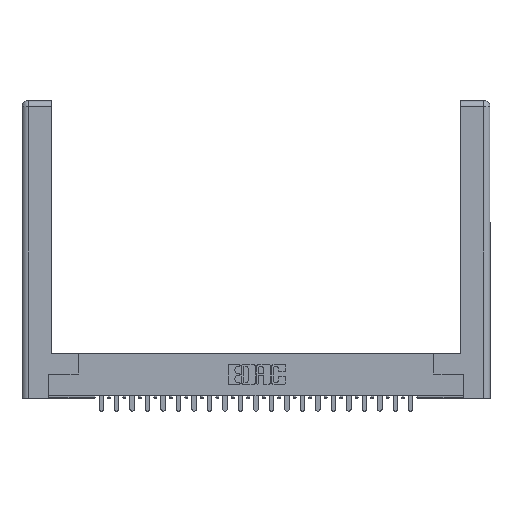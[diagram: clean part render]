
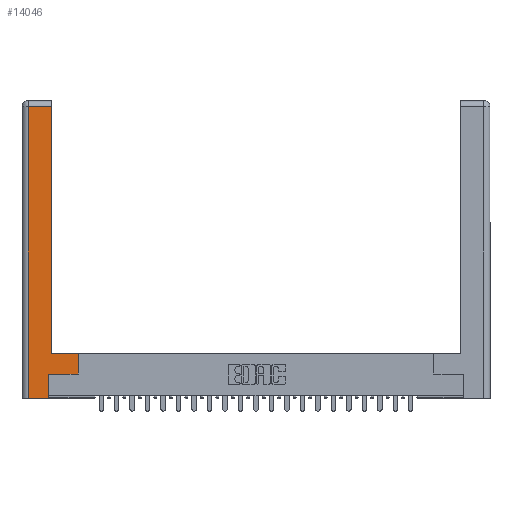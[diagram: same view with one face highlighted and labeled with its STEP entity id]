
A CAD part, top view. The second image highlights one B-rep face of the part: STEP entity #14046.
In plain terms, the highlighted planar face has unit normal (0, 0, 1).
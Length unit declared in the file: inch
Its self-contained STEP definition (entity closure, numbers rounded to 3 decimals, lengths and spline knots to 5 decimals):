
#110 = CARTESIAN_POINT ( 'NONE',  ( 0.265, 0., 0. ) ) ;
#806 = CARTESIAN_POINT ( 'NONE',  ( 0.295, 0.45, 0. ) ) ;
#1246 = ORIENTED_EDGE ( 'NONE', *, *, #8433, .T. ) ;
#1459 = DIRECTION ( 'NONE',  ( 0., 1., 0. ) ) ;
#1823 = VECTOR ( 'NONE', #17941, 39.37008 ) ;
#2029 = EDGE_CURVE ( 'NONE', #27252, #5921, #13883, .T. ) ;
#2467 = EDGE_CURVE ( 'NONE', #15852, #5702, #19233, .T. ) ;
#2565 = VECTOR ( 'NONE', #17261, 39.37008 ) ;
#3024 = EDGE_CURVE ( 'NONE', #6305, #15852, #15585, .T. ) ;
#3423 = VECTOR ( 'NONE', #1459, 39.37008 ) ;
#3625 = PLANE ( 'NONE',  #19880 ) ;
#3725 = CARTESIAN_POINT ( 'NONE',  ( 0., 0., 0. ) ) ;
#4234 = CARTESIAN_POINT ( 'NONE',  ( 0.295, 0.45, 0. ) ) ;
#4436 = DIRECTION ( 'NONE',  ( 0., 1., 0. ) ) ;
#4455 = LINE ( 'NONE', #6369, #21232 ) ;
#4525 = CARTESIAN_POINT ( 'NONE',  ( 0.265, 0., 0. ) ) ;
#5032 = CARTESIAN_POINT ( 'NONE',  ( 0.565, 0.245, 0. ) ) ;
#5157 = CARTESIAN_POINT ( 'NONE',  ( 0.565, 0.45, 0. ) ) ;
#5620 = CARTESIAN_POINT ( 'NONE',  ( 0.265, 0.245, 0. ) ) ;
#5702 = VERTEX_POINT ( 'NONE', #5620 ) ;
#5921 = VERTEX_POINT ( 'NONE', #4234 ) ;
#6305 = VERTEX_POINT ( 'NONE', #24982 ) ;
#6361 = DIRECTION ( 'NONE',  ( 1., 0., 0. ) ) ;
#6369 = CARTESIAN_POINT ( 'NONE',  ( 0.295, 3., 0. ) ) ;
#8200 = DIRECTION ( 'NONE',  ( -1., 0., 0. ) ) ;
#8433 = EDGE_CURVE ( 'NONE', #16496, #6305, #26839, .T. ) ;
#8666 = ORIENTED_EDGE ( 'NONE', *, *, #2029, .T. ) ;
#8725 = DIRECTION ( 'NONE',  ( 1., 0., 0. ) ) ;
#9006 = EDGE_CURVE ( 'NONE', #5702, #26140, #17341, .T. ) ;
#9168 = FACE_OUTER_BOUND ( 'NONE', #19815, .T. ) ;
#9353 = VERTEX_POINT ( 'NONE', #16063 ) ;
#10586 = LINE ( 'NONE', #27814, #2565 ) ;
#11407 = ORIENTED_EDGE ( 'NONE', *, *, #3024, .T. ) ;
#13883 = LINE ( 'NONE', #806, #1823 ) ;
#14046 = ADVANCED_FACE ( 'NONE', ( #9168 ), #3625, .F. ) ;
#14267 = CARTESIAN_POINT ( 'NONE',  ( 0.565, 0.45, 0. ) ) ;
#14525 = ORIENTED_EDGE ( 'NONE', *, *, #26291, .T. ) ;
#15132 = LINE ( 'NONE', #14267, #3423 ) ;
#15585 = LINE ( 'NONE', #4525, #22001 ) ;
#15852 = VERTEX_POINT ( 'NONE', #110 ) ;
#16063 = CARTESIAN_POINT ( 'NONE',  ( 0.295, 2.94, 0. ) ) ;
#16193 = VECTOR ( 'NONE', #4436, 39.37008 ) ;
#16253 = CARTESIAN_POINT ( 'NONE',  ( 0.0615, 0., 0. ) ) ;
#16496 = VERTEX_POINT ( 'NONE', #20030 ) ;
#17261 = DIRECTION ( 'NONE',  ( -1., 0., 0. ) ) ;
#17341 = LINE ( 'NONE', #27676, #26801 ) ;
#17399 = ORIENTED_EDGE ( 'NONE', *, *, #2467, .T. ) ;
#17941 = DIRECTION ( 'NONE',  ( -1., 0., 0. ) ) ;
#19059 = CARTESIAN_POINT ( 'NONE',  ( 0.265, 0.245, 0. ) ) ;
#19233 = LINE ( 'NONE', #19059, #16193 ) ;
#19392 = EDGE_CURVE ( 'NONE', #9353, #16496, #10586, .T. ) ;
#19815 = EDGE_LOOP ( 'NONE', ( #20419, #23531, #1246, #11407, #17399, #24002, #14525, #8666 ) ) ;
#19880 = AXIS2_PLACEMENT_3D ( 'NONE', #3725, #21078, #8200 ) ;
#20030 = CARTESIAN_POINT ( 'NONE',  ( 0.0615, 2.94, 0. ) ) ;
#20419 = ORIENTED_EDGE ( 'NONE', *, *, #25803, .T. ) ;
#21078 = DIRECTION ( 'NONE',  ( 0., 0., -1. ) ) ;
#21232 = VECTOR ( 'NONE', #21386, 39.37008 ) ;
#21386 = DIRECTION ( 'NONE',  ( 0., 1., 0. ) ) ;
#22001 = VECTOR ( 'NONE', #8725, 39.37008 ) ;
#22405 = DIRECTION ( 'NONE',  ( 0., -1., 0. ) ) ;
#23531 = ORIENTED_EDGE ( 'NONE', *, *, #19392, .T. ) ;
#24002 = ORIENTED_EDGE ( 'NONE', *, *, #9006, .T. ) ;
#24512 = VECTOR ( 'NONE', #22405, 39.37008 ) ;
#24982 = CARTESIAN_POINT ( 'NONE',  ( 0.0615, 0., 0. ) ) ;
#25803 = EDGE_CURVE ( 'NONE', #5921, #9353, #4455, .T. ) ;
#26140 = VERTEX_POINT ( 'NONE', #5032 ) ;
#26291 = EDGE_CURVE ( 'NONE', #26140, #27252, #15132, .T. ) ;
#26801 = VECTOR ( 'NONE', #6361, 39.37008 ) ;
#26839 = LINE ( 'NONE', #16253, #24512 ) ;
#27252 = VERTEX_POINT ( 'NONE', #5157 ) ;
#27676 = CARTESIAN_POINT ( 'NONE',  ( 0.565, 0.245, 0. ) ) ;
#27814 = CARTESIAN_POINT ( 'NONE',  ( 0.0615, 2.94, 0. ) ) ;
